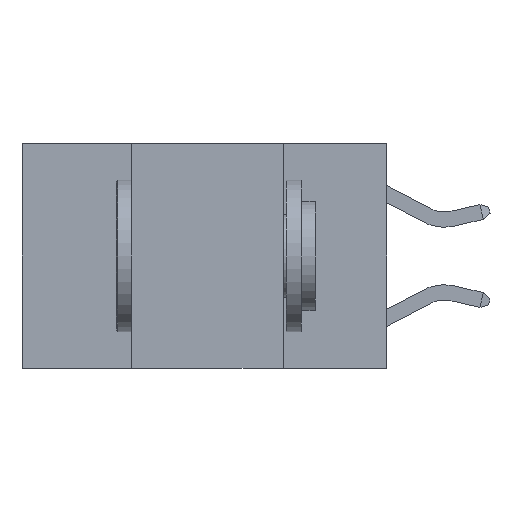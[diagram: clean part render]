
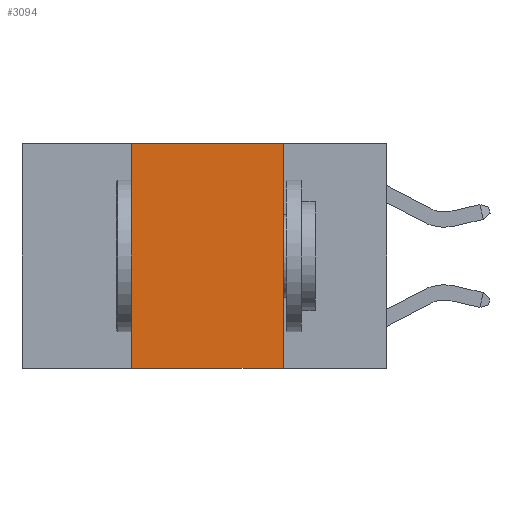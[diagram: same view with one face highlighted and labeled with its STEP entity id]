
A CAD part, left-side view. The second image highlights one B-rep face of the part: STEP entity #3094.
In plain terms, the highlighted planar face has unit normal (-1, 0, 0).
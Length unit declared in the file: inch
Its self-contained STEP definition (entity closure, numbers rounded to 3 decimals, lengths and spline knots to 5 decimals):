
#73 = DIRECTION ( 'NONE',  ( 0., 0., 1. ) ) ;
#523 = CARTESIAN_POINT ( 'NONE',  ( 0., 0.42, -0.37 ) ) ;
#580 = CARTESIAN_POINT ( 'NONE',  ( 0., 0.17, 0. ) ) ;
#692 = LINE ( 'NONE', #1620, #8505 ) ;
#1379 = DIRECTION ( 'NONE',  ( 1., 0., 0. ) ) ;
#1503 = DIRECTION ( 'NONE',  ( 0., -1., 0. ) ) ;
#1620 = CARTESIAN_POINT ( 'NONE',  ( 0., 0.6, 0. ) ) ;
#1864 = VECTOR ( 'NONE', #73, 39.37008 ) ;
#2147 = ORIENTED_EDGE ( 'NONE', *, *, #7773, .T. ) ;
#2932 = ORIENTED_EDGE ( 'NONE', *, *, #10235, .F. ) ;
#3094 = ADVANCED_FACE ( 'NONE', ( #5474 ), #6272, .F. ) ;
#3628 = DIRECTION ( 'NONE',  ( 0., -1., 0. ) ) ;
#4494 = ORIENTED_EDGE ( 'NONE', *, *, #5305, .F. ) ;
#4595 = ORIENTED_EDGE ( 'NONE', *, *, #8475, .F. ) ;
#4657 = VECTOR ( 'NONE', #3628, 39.37008 ) ;
#5305 = EDGE_CURVE ( 'NONE', #6059, #8232, #692, .T. ) ;
#5474 = FACE_OUTER_BOUND ( 'NONE', #7543, .T. ) ;
#5507 = VECTOR ( 'NONE', #5641, 39.37008 ) ;
#5524 = CARTESIAN_POINT ( 'NONE',  ( 0., 0.6, 0. ) ) ;
#5641 = DIRECTION ( 'NONE',  ( 0., 0., -1. ) ) ;
#6059 = VERTEX_POINT ( 'NONE', #6909 ) ;
#6272 = PLANE ( 'NONE',  #6992 ) ;
#6909 = CARTESIAN_POINT ( 'NONE',  ( 0., 0.42, 0. ) ) ;
#6992 = AXIS2_PLACEMENT_3D ( 'NONE', #5524, #1379, #8865 ) ;
#7062 = VERTEX_POINT ( 'NONE', #523 ) ;
#7209 = CARTESIAN_POINT ( 'NONE',  ( 0., 0.17, -0.37 ) ) ;
#7543 = EDGE_LOOP ( 'NONE', ( #4595, #4494, #2932, #2147 ) ) ;
#7580 = CARTESIAN_POINT ( 'NONE',  ( 0., 0.17, 0. ) ) ;
#7687 = LINE ( 'NONE', #9325, #4657 ) ;
#7773 = EDGE_CURVE ( 'NONE', #7062, #10590, #7687, .T. ) ;
#8232 = VERTEX_POINT ( 'NONE', #7580 ) ;
#8475 = EDGE_CURVE ( 'NONE', #8232, #10590, #9619, .T. ) ;
#8505 = VECTOR ( 'NONE', #1503, 39.37008 ) ;
#8865 = DIRECTION ( 'NONE',  ( 0., 0., -1. ) ) ;
#9232 = LINE ( 'NONE', #10699, #1864 ) ;
#9325 = CARTESIAN_POINT ( 'NONE',  ( 0., 0.6, -0.37 ) ) ;
#9619 = LINE ( 'NONE', #580, #5507 ) ;
#10235 = EDGE_CURVE ( 'NONE', #7062, #6059, #9232, .T. ) ;
#10590 = VERTEX_POINT ( 'NONE', #7209 ) ;
#10699 = CARTESIAN_POINT ( 'NONE',  ( 0., 0.42, 0. ) ) ;
